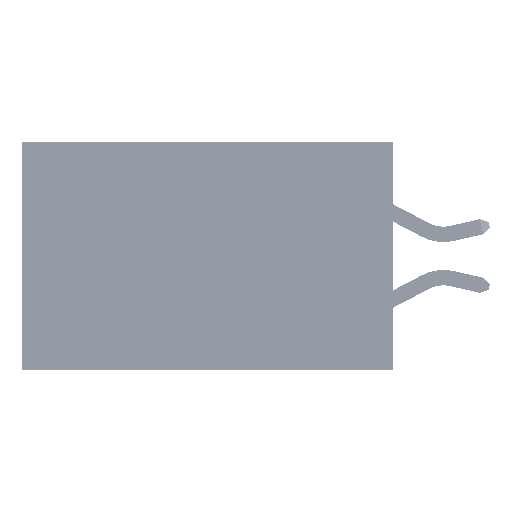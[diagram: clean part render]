
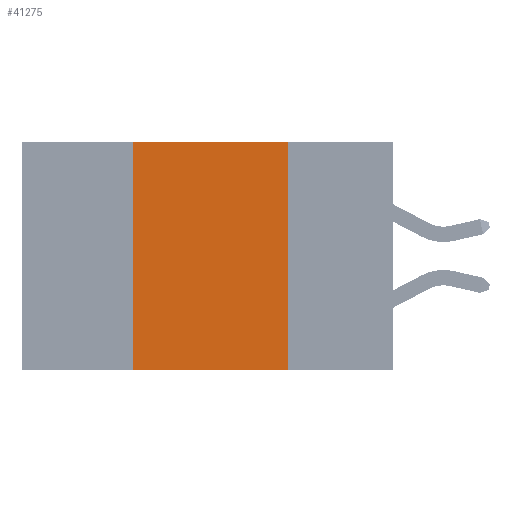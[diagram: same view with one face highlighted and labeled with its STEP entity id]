
A CAD part, left-side view. The second image highlights one B-rep face of the part: STEP entity #41275.
In plain terms, the highlighted planar face has unit normal (-1, 0, 0).
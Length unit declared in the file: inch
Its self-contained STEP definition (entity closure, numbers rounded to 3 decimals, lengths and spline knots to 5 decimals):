
#3088 = EDGE_CURVE ( 'NONE', #50785, #47900, #31516, .T. ) ;
#3493 = CARTESIAN_POINT ( 'NONE',  ( 0., 0.6, 0. ) ) ;
#7472 = FACE_OUTER_BOUND ( 'NONE', #49188, .T. ) ;
#7851 = LINE ( 'NONE', #16897, #29366 ) ;
#8435 = VECTOR ( 'NONE', #38990, 39.37008 ) ;
#11282 = CARTESIAN_POINT ( 'NONE',  ( 0., 0.17, -0.37 ) ) ;
#11633 = ORIENTED_EDGE ( 'NONE', *, *, #40287, .F. ) ;
#11726 = DIRECTION ( 'NONE',  ( 0., 0., -1. ) ) ;
#12008 = VECTOR ( 'NONE', #45923, 39.37008 ) ;
#12520 = EDGE_CURVE ( 'NONE', #21748, #42001, #50183, .T. ) ;
#14461 = ORIENTED_EDGE ( 'NONE', *, *, #3088, .F. ) ;
#14949 = CARTESIAN_POINT ( 'NONE',  ( 0., 0.42, 0. ) ) ;
#16897 = CARTESIAN_POINT ( 'NONE',  ( 0., 0.6, 0. ) ) ;
#19895 = CARTESIAN_POINT ( 'NONE',  ( 0., 0.6, -0.37 ) ) ;
#21748 = VERTEX_POINT ( 'NONE', #44069 ) ;
#23977 = CARTESIAN_POINT ( 'NONE',  ( 0., 0.42, -0.37 ) ) ;
#24361 = DIRECTION ( 'NONE',  ( 0., -1., 0. ) ) ;
#26752 = CARTESIAN_POINT ( 'NONE',  ( 0., 0.42, 0. ) ) ;
#28636 = VECTOR ( 'NONE', #48147, 39.37008 ) ;
#29366 = VECTOR ( 'NONE', #24361, 39.37008 ) ;
#29647 = CARTESIAN_POINT ( 'NONE',  ( 0., 0.17, 0. ) ) ;
#31516 = LINE ( 'NONE', #26752, #8435 ) ;
#38990 = DIRECTION ( 'NONE',  ( 0., 0., 1. ) ) ;
#39948 = PLANE ( 'NONE',  #48058 ) ;
#40287 = EDGE_CURVE ( 'NONE', #47900, #21748, #7851, .T. ) ;
#41275 = ADVANCED_FACE ( 'NONE', ( #7472 ), #39948, .F. ) ;
#42001 = VERTEX_POINT ( 'NONE', #11282 ) ;
#42259 = ORIENTED_EDGE ( 'NONE', *, *, #12520, .F. ) ;
#44069 = CARTESIAN_POINT ( 'NONE',  ( 0., 0.17, 0. ) ) ;
#45923 = DIRECTION ( 'NONE',  ( 0., 0., -1. ) ) ;
#47900 = VERTEX_POINT ( 'NONE', #14949 ) ;
#47992 = ORIENTED_EDGE ( 'NONE', *, *, #48051, .T. ) ;
#48051 = EDGE_CURVE ( 'NONE', #50785, #42001, #50644, .T. ) ;
#48058 = AXIS2_PLACEMENT_3D ( 'NONE', #3493, #48225, #11726 ) ;
#48147 = DIRECTION ( 'NONE',  ( 0., -1., 0. ) ) ;
#48225 = DIRECTION ( 'NONE',  ( 1., 0., 0. ) ) ;
#49188 = EDGE_LOOP ( 'NONE', ( #42259, #11633, #14461, #47992 ) ) ;
#50183 = LINE ( 'NONE', #29647, #12008 ) ;
#50644 = LINE ( 'NONE', #19895, #28636 ) ;
#50785 = VERTEX_POINT ( 'NONE', #23977 ) ;
